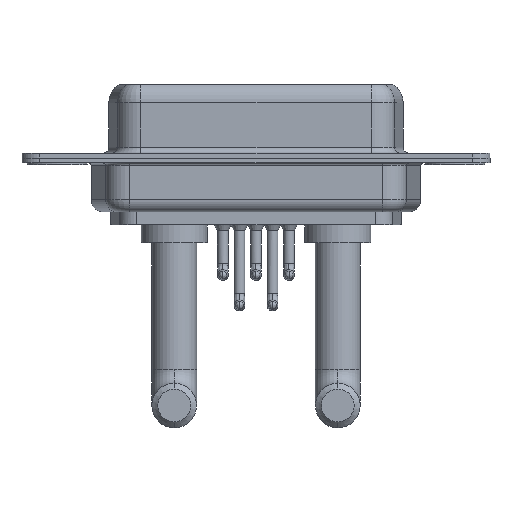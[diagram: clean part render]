
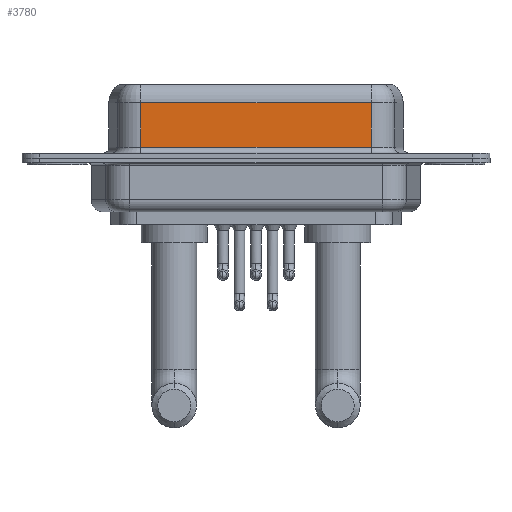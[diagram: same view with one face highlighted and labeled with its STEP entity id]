
A CAD part, front view. The second image highlights one B-rep face of the part: STEP entity #3780.
In plain terms, the highlighted planar face has unit normal (0, -1, 0).
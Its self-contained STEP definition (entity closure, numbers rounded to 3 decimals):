
#286 = LINE ( 'NONE', #2951, #1233 ) ;
#1000 = LINE ( 'NONE', #4422, #13438 ) ;
#1010 = ORIENTED_EDGE ( 'NONE', *, *, #8180, .T. ) ;
#1233 = VECTOR ( 'NONE', #6313, 1000. ) ;
#1362 = EDGE_LOOP ( 'NONE', ( #10891, #1010, #10494, #3627 ) ) ;
#1656 = CARTESIAN_POINT ( 'NONE',  ( 7.013, -3.95, 4.65 ) ) ;
#1821 = DIRECTION ( 'NONE',  ( 0., 0., 1. ) ) ;
#2406 = CARTESIAN_POINT ( 'NONE',  ( 7.013, -3.95, 0.9 ) ) ;
#2951 = CARTESIAN_POINT ( 'NONE',  ( 7.013, -3.95, 6.4 ) ) ;
#3627 = ORIENTED_EDGE ( 'NONE', *, *, #15015, .T. ) ;
#3780 = ADVANCED_FACE ( 'NONE', ( #8766 ), #10967, .F. ) ;
#4050 = VECTOR ( 'NONE', #5770, 1000. ) ;
#4422 = CARTESIAN_POINT ( 'NONE',  ( 26.287, -3.95, 4.65 ) ) ;
#4546 = LINE ( 'NONE', #14944, #4050 ) ;
#4591 = VERTEX_POINT ( 'NONE', #2406 ) ;
#5104 = VERTEX_POINT ( 'NONE', #5483 ) ;
#5483 = CARTESIAN_POINT ( 'NONE',  ( 26.287, -3.95, 0.9 ) ) ;
#5646 = AXIS2_PLACEMENT_3D ( 'NONE', #8846, #13359, #1821 ) ;
#5770 = DIRECTION ( 'NONE',  ( 0., 0., -1. ) ) ;
#6313 = DIRECTION ( 'NONE',  ( 0., 0., -1. ) ) ;
#6812 = DIRECTION ( 'NONE',  ( -1., 0., 0. ) ) ;
#8180 = EDGE_CURVE ( 'NONE', #13435, #11414, #1000, .T. ) ;
#8283 = EDGE_CURVE ( 'NONE', #11414, #4591, #286, .T. ) ;
#8766 = FACE_OUTER_BOUND ( 'NONE', #1362, .T. ) ;
#8846 = CARTESIAN_POINT ( 'NONE',  ( 26.287, -3.95, 6.4 ) ) ;
#9137 = VECTOR ( 'NONE', #13743, 1000. ) ;
#9145 = LINE ( 'NONE', #9219, #9137 ) ;
#9219 = CARTESIAN_POINT ( 'NONE',  ( 26.287, -3.95, 0.9 ) ) ;
#10494 = ORIENTED_EDGE ( 'NONE', *, *, #8283, .T. ) ;
#10891 = ORIENTED_EDGE ( 'NONE', *, *, #14226, .F. ) ;
#10967 = PLANE ( 'NONE',  #5646 ) ;
#11414 = VERTEX_POINT ( 'NONE', #1656 ) ;
#11985 = CARTESIAN_POINT ( 'NONE',  ( 26.287, -3.95, 4.65 ) ) ;
#13359 = DIRECTION ( 'NONE',  ( 0., 1., 0. ) ) ;
#13435 = VERTEX_POINT ( 'NONE', #11985 ) ;
#13438 = VECTOR ( 'NONE', #6812, 1000. ) ;
#13743 = DIRECTION ( 'NONE',  ( 1., 0., 0. ) ) ;
#14226 = EDGE_CURVE ( 'NONE', #13435, #5104, #4546, .T. ) ;
#14944 = CARTESIAN_POINT ( 'NONE',  ( 26.287, -3.95, 6.4 ) ) ;
#15015 = EDGE_CURVE ( 'NONE', #4591, #5104, #9145, .T. ) ;
